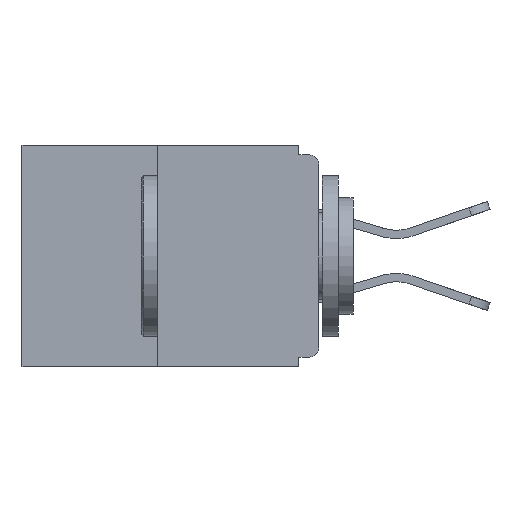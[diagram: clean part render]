
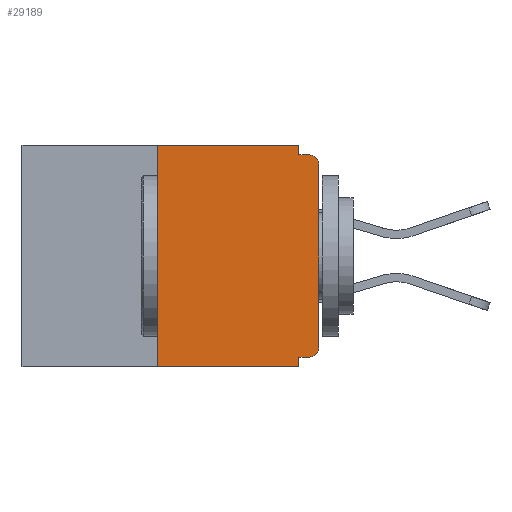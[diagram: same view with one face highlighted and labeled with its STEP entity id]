
A CAD part, left-side view. The second image highlights one B-rep face of the part: STEP entity #29189.
In plain terms, the highlighted planar face has unit normal (-1, 0, 0).
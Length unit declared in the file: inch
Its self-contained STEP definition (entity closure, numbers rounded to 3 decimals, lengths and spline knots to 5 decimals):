
#751 = CARTESIAN_POINT ( 'NONE',  ( 0., 0.031, -0.015 ) ) ;
#916 = ORIENTED_EDGE ( 'NONE', *, *, #25012, .T. ) ;
#1004 = AXIS2_PLACEMENT_3D ( 'NONE', #5373, #22332, #5587 ) ;
#1228 = LINE ( 'NONE', #25173, #6448 ) ;
#1590 = CARTESIAN_POINT ( 'NONE',  ( 0., 0.25, -0.343 ) ) ;
#1681 = PLANE ( 'NONE',  #29173 ) ;
#1731 = CIRCLE ( 'NONE', #1004, 0.015 ) ;
#1801 = LINE ( 'NONE', #25927, #22652 ) ;
#2345 = ORIENTED_EDGE ( 'NONE', *, *, #19668, .T. ) ;
#2504 = LINE ( 'NONE', #7973, #24465 ) ;
#2597 = LINE ( 'NONE', #6035, #30138 ) ;
#2829 = VERTEX_POINT ( 'NONE', #3367 ) ;
#3367 = CARTESIAN_POINT ( 'NONE',  ( 0., 0.015, -0.015 ) ) ;
#3444 = CARTESIAN_POINT ( 'NONE',  ( 0., 0.031, -0.343 ) ) ;
#3656 = LINE ( 'NONE', #30276, #21527 ) ;
#4718 = VECTOR ( 'NONE', #20761, 39.37008 ) ;
#4746 = FACE_OUTER_BOUND ( 'NONE', #21758, .T. ) ;
#5330 = EDGE_CURVE ( 'NONE', #22071, #16423, #2504, .T. ) ;
#5373 = CARTESIAN_POINT ( 'NONE',  ( 0., 0.015, -0.03 ) ) ;
#5587 = DIRECTION ( 'NONE',  ( 0., 0., -1. ) ) ;
#5828 = CARTESIAN_POINT ( 'NONE',  ( 0., 0.015, -0.328 ) ) ;
#5984 = DIRECTION ( 'NONE',  ( -1., 0., 0. ) ) ;
#6035 = CARTESIAN_POINT ( 'NONE',  ( 0., 0.46, -0.343 ) ) ;
#6158 = DIRECTION ( 'NONE',  ( 0., 0., -1. ) ) ;
#6430 = ORIENTED_EDGE ( 'NONE', *, *, #20340, .F. ) ;
#6448 = VECTOR ( 'NONE', #10918, 39.37008 ) ;
#6581 = VERTEX_POINT ( 'NONE', #28027 ) ;
#7973 = CARTESIAN_POINT ( 'NONE',  ( 0., 0.25, 0. ) ) ;
#8461 = LINE ( 'NONE', #8592, #4718 ) ;
#8592 = CARTESIAN_POINT ( 'NONE',  ( 0., 0.031, 0. ) ) ;
#8678 = DIRECTION ( 'NONE',  ( 0., 0., -1. ) ) ;
#9473 = CARTESIAN_POINT ( 'NONE',  ( 0., 0.031, -0.343 ) ) ;
#9573 = CARTESIAN_POINT ( 'NONE',  ( 0., 0.46, 0. ) ) ;
#9639 = LINE ( 'NONE', #9573, #27909 ) ;
#10327 = ORIENTED_EDGE ( 'NONE', *, *, #21743, .F. ) ;
#10918 = DIRECTION ( 'NONE',  ( 0., 0., 1. ) ) ;
#11035 = DIRECTION ( 'NONE',  ( 1., 0., 0. ) ) ;
#11154 = EDGE_CURVE ( 'NONE', #17828, #30768, #3656, .T. ) ;
#11544 = DIRECTION ( 'NONE',  ( 0., -1., 0. ) ) ;
#11854 = DIRECTION ( 'NONE',  ( 0., -1., 0. ) ) ;
#12496 = VERTEX_POINT ( 'NONE', #3444 ) ;
#12913 = DIRECTION ( 'NONE',  ( 0., 1., 0. ) ) ;
#12960 = ORIENTED_EDGE ( 'NONE', *, *, #5330, .F. ) ;
#13205 = CARTESIAN_POINT ( 'NONE',  ( 0., 0.031, -0.328 ) ) ;
#13716 = EDGE_CURVE ( 'NONE', #6581, #20376, #1228, .T. ) ;
#15051 = VERTEX_POINT ( 'NONE', #751 ) ;
#15920 = VECTOR ( 'NONE', #18637, 39.37008 ) ;
#16052 = EDGE_CURVE ( 'NONE', #16423, #27362, #9639, .T. ) ;
#16423 = VERTEX_POINT ( 'NONE', #27372 ) ;
#16700 = ORIENTED_EDGE ( 'NONE', *, *, #16052, .F. ) ;
#16735 = AXIS2_PLACEMENT_3D ( 'NONE', #20238, #5984, #8678 ) ;
#17828 = VERTEX_POINT ( 'NONE', #5828 ) ;
#18637 = DIRECTION ( 'NONE',  ( 0., 0., -1. ) ) ;
#18843 = CARTESIAN_POINT ( 'NONE',  ( 0., 0., -0.03 ) ) ;
#19668 = EDGE_CURVE ( 'NONE', #22071, #12496, #2597, .T. ) ;
#20238 = CARTESIAN_POINT ( 'NONE',  ( 0., 0.015, -0.313 ) ) ;
#20334 = EDGE_CURVE ( 'NONE', #30768, #12496, #28934, .T. ) ;
#20340 = EDGE_CURVE ( 'NONE', #15051, #2829, #1801, .T. ) ;
#20376 = VERTEX_POINT ( 'NONE', #18843 ) ;
#20761 = DIRECTION ( 'NONE',  ( 0., 0., -1. ) ) ;
#21230 = ORIENTED_EDGE ( 'NONE', *, *, #11154, .F. ) ;
#21519 = ORIENTED_EDGE ( 'NONE', *, *, #23858, .T. ) ;
#21527 = VECTOR ( 'NONE', #12913, 39.37008 ) ;
#21743 = EDGE_CURVE ( 'NONE', #27362, #15051, #8461, .T. ) ;
#21758 = EDGE_LOOP ( 'NONE', ( #16700, #12960, #2345, #22182, #21230, #916, #28405, #21519, #6430, #10327 ) ) ;
#22071 = VERTEX_POINT ( 'NONE', #1590 ) ;
#22182 = ORIENTED_EDGE ( 'NONE', *, *, #20334, .F. ) ;
#22252 = DIRECTION ( 'NONE',  ( 0., 0., 1. ) ) ;
#22332 = DIRECTION ( 'NONE',  ( -1., 0., 0. ) ) ;
#22652 = VECTOR ( 'NONE', #11544, 39.37008 ) ;
#23183 = CARTESIAN_POINT ( 'NONE',  ( 0., 0.031, 0. ) ) ;
#23858 = EDGE_CURVE ( 'NONE', #20376, #2829, #1731, .T. ) ;
#24465 = VECTOR ( 'NONE', #22252, 39.37008 ) ;
#25012 = EDGE_CURVE ( 'NONE', #17828, #6581, #25842, .T. ) ;
#25173 = CARTESIAN_POINT ( 'NONE',  ( 0., 0., 0. ) ) ;
#25303 = CARTESIAN_POINT ( 'NONE',  ( 0., 0.46, 0. ) ) ;
#25842 = CIRCLE ( 'NONE', #16735, 0.015 ) ;
#25927 = CARTESIAN_POINT ( 'NONE',  ( 0., 0., -0.015 ) ) ;
#27362 = VERTEX_POINT ( 'NONE', #23183 ) ;
#27372 = CARTESIAN_POINT ( 'NONE',  ( 0., 0.25, 0. ) ) ;
#27909 = VECTOR ( 'NONE', #11854, 39.37008 ) ;
#28027 = CARTESIAN_POINT ( 'NONE',  ( 0., 0., -0.313 ) ) ;
#28405 = ORIENTED_EDGE ( 'NONE', *, *, #13716, .T. ) ;
#28934 = LINE ( 'NONE', #9473, #15920 ) ;
#29173 = AXIS2_PLACEMENT_3D ( 'NONE', #25303, #11035, #6158 ) ;
#29189 = ADVANCED_FACE ( 'NONE', ( #4746 ), #1681, .F. ) ;
#29936 = DIRECTION ( 'NONE',  ( 0., -1., 0. ) ) ;
#30138 = VECTOR ( 'NONE', #29936, 39.37008 ) ;
#30276 = CARTESIAN_POINT ( 'NONE',  ( 0., 0., -0.328 ) ) ;
#30768 = VERTEX_POINT ( 'NONE', #13205 ) ;
